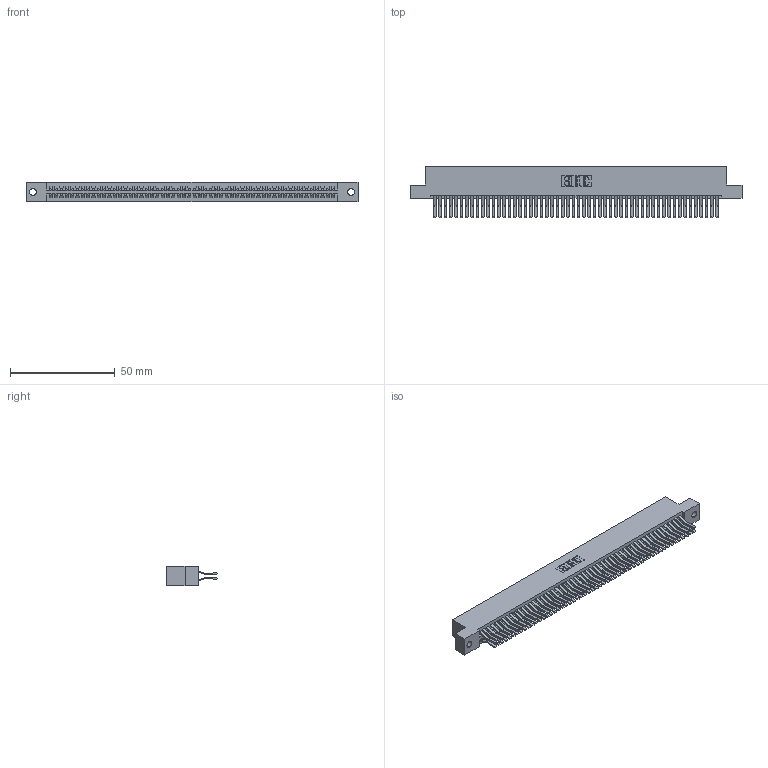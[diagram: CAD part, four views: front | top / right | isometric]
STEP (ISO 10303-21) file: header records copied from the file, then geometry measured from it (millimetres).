
FILE_DESCRIPTION (( 'STEP AP203' ), '1' );
FILE_NAME ('395-108-560-202.STEP', '2018-12-01T00:40:52', ( '' ), ( '' ), 'SwSTEP 2.0', 'SolidWorks 2016', '' );
FILE_SCHEMA (( 'CONFIG_CONTROL_DESIGN' ));
Length unit declared in the file: inch
Products named in the file (3): 345-292-001_560 Tail; 395-108-560-202; 345 Part_Flush Mounting Lugs - 0.128 Dia
Assembly tree (109 placements, depth 2):
  395-108-560-202
    345 Part_Flush Mounting Lugs - 0.128 Dia
    345-292-001_560 Tail  x108
Bounding box: 158.37 x 24.45 x 9.4 mm (x, y, z)
Volume: 16166.7 mm3; surface area: 25677.5 mm2
Topology: 109 solids, 109 shells, 5742 faces, 17081 edges, 11242 vertices
Faces by surface type: plane 3644, cylinder 2098
Entity records: 40845 total; most frequent: CARTESIAN_POINT 6836, ORIENTED_EDGE 6770, DIRECTION 6017, EDGE_CURVE 3385, VECTOR 3033, LINE 3033, VERTEX_POINT 2254, AXIS2_PLACEMENT_3D 1492
